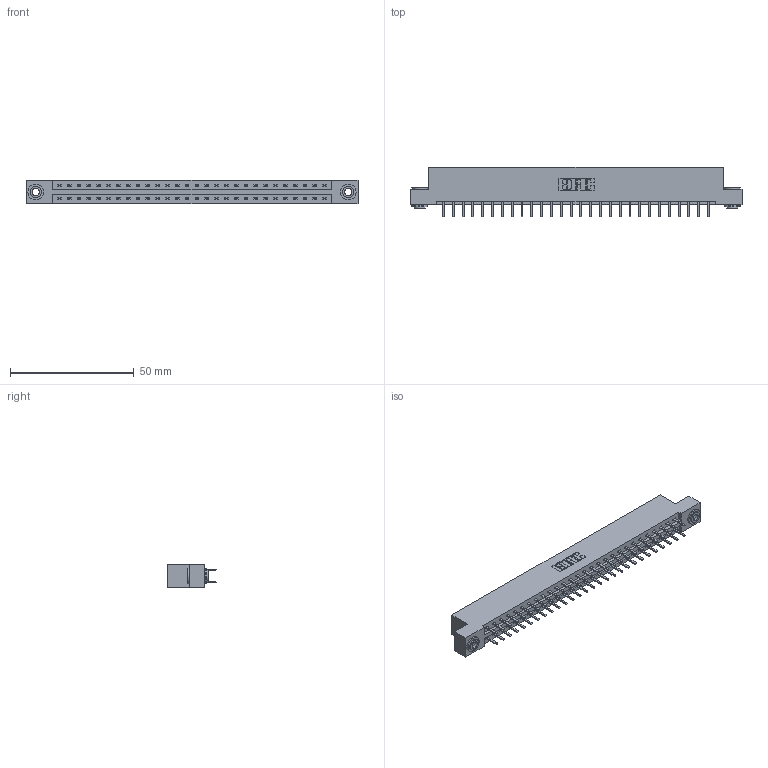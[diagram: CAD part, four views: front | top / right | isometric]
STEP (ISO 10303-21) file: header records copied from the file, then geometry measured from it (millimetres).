
FILE_DESCRIPTION (( 'STEP AP203' ), '1' );
FILE_NAME ('337-056-520-203.STEP', '2019-10-09T18:46:54', ( '' ), ( '' ), 'SwSTEP 2.0', 'SolidWorks 2016', '' );
FILE_SCHEMA (( 'CONFIG_CONTROL_DESIGN' ));
Length unit declared in the file: inch
Products named in the file (4): 345-292-001_345-293-120; 337-056-520-203; 337 Part_Flush Mounting Lugs - 0.156 Dia-TH; 345-250-002_345-250-002-102
Assembly tree (59 placements, depth 2):
  337-056-520-203
    337 Part_Flush Mounting Lugs - 0.156 Dia-TH
    345-292-001_345-293-120  x56
    345-250-002_345-250-002-102  x2
Bounding box: 133.96 x 20.02 x 9.4 mm (x, y, z)
Volume: 13926.1 mm3; surface area: 15761.7 mm2
Topology: 59 solids, 59 shells, 3400 faces, 9851 edges, 6414 vertices
Faces by surface type: plane 2320, cylinder 1072, cone 8
Entity records: 24284 total; most frequent: CARTESIAN_POINT 4089, ORIENTED_EDGE 4006, DIRECTION 3525, EDGE_CURVE 2003, VECTOR 1847, LINE 1847, VERTEX_POINT 1330, AXIS2_PLACEMENT_3D 839
